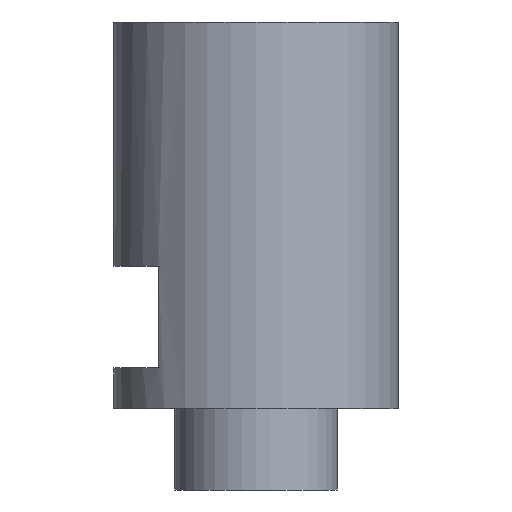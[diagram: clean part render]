
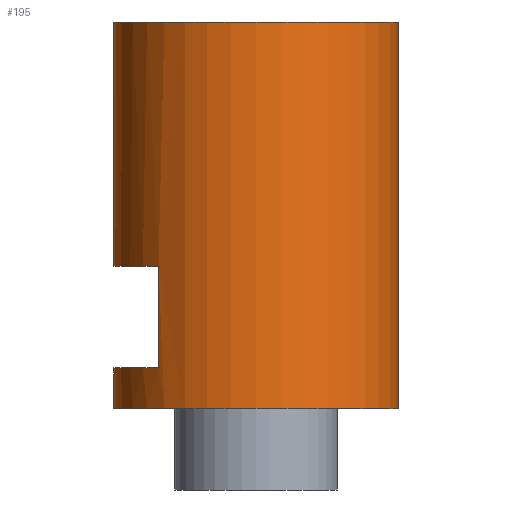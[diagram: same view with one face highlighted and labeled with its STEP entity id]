
A CAD part, front view. The second image highlights one B-rep face of the part: STEP entity #195.
In plain terms, the highlighted cylindrical face has radius 7 mm (diameter 14 mm), a partial arc.
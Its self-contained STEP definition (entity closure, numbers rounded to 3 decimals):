
#3 = CIRCLE ( 'NONE', #515, 7. ) ;
#4 = ORIENTED_EDGE ( 'NONE', *, *, #141, .T. ) ;
#9 = ORIENTED_EDGE ( 'NONE', *, *, #354, .F. ) ;
#28 = DIRECTION ( 'NONE',  ( 1., 0., 0. ) ) ;
#29 = CIRCLE ( 'NONE', #196, 7. ) ;
#32 = VERTEX_POINT ( 'NONE', #520 ) ;
#38 = LINE ( 'NONE', #447, #513 ) ;
#43 = DIRECTION ( 'NONE',  ( 0., 0., -1. ) ) ;
#45 = CARTESIAN_POINT ( 'NONE',  ( 0., 0., 19. ) ) ;
#50 = AXIS2_PLACEMENT_3D ( 'NONE', #122, #299, #28 ) ;
#58 = ORIENTED_EDGE ( 'NONE', *, *, #287, .T. ) ;
#71 = DIRECTION ( 'NONE',  ( 0., 0., -1. ) ) ;
#73 = DIRECTION ( 'NONE',  ( 0., 0., -1. ) ) ;
#80 = CARTESIAN_POINT ( 'NONE',  ( -7., 0., 6. ) ) ;
#88 = EDGE_CURVE ( 'NONE', #245, #32, #222, .T. ) ;
#93 = VERTEX_POINT ( 'NONE', #264 ) ;
#96 = EDGE_LOOP ( 'NONE', ( #385, #9, #58, #238, #387, #536, #4, #511 ) ) ;
#99 = FACE_OUTER_BOUND ( 'NONE', #96, .T. ) ;
#111 = VECTOR ( 'NONE', #73, 1000. ) ;
#121 = EDGE_CURVE ( 'NONE', #168, #93, #156, .T. ) ;
#122 = CARTESIAN_POINT ( 'NONE',  ( 0., 0., 7. ) ) ;
#134 = CYLINDRICAL_SURFACE ( 'NONE', #166, 7. ) ;
#141 = EDGE_CURVE ( 'NONE', #479, #410, #38, .T. ) ;
#143 = AXIS2_PLACEMENT_3D ( 'NONE', #459, #551, #228 ) ;
#156 = LINE ( 'NONE', #203, #111 ) ;
#166 = AXIS2_PLACEMENT_3D ( 'NONE', #529, #396, #581 ) ;
#168 = VERTEX_POINT ( 'NONE', #348 ) ;
#172 = VECTOR ( 'NONE', #43, 1000. ) ;
#180 = DIRECTION ( 'NONE',  ( 1., 0., 0. ) ) ;
#189 = LINE ( 'NONE', #80, #172 ) ;
#190 = DIRECTION ( 'NONE',  ( 0., 0., -1. ) ) ;
#195 = ADVANCED_FACE ( 'NONE', ( #99 ), #134, .T. ) ;
#196 = AXIS2_PLACEMENT_3D ( 'NONE', #45, #317, #180 ) ;
#203 = CARTESIAN_POINT ( 'NONE',  ( 7., 0., 6. ) ) ;
#212 = EDGE_CURVE ( 'NONE', #479, #487, #3, .T. ) ;
#222 = CIRCLE ( 'NONE', #50, 7. ) ;
#221 = CARTESIAN_POINT ( 'NONE',  ( 0., 0., 2. ) ) ;
#228 = DIRECTION ( 'NONE',  ( 1., 0., 0. ) ) ;
#238 = ORIENTED_EDGE ( 'NONE', *, *, #88, .T. ) ;
#243 = VECTOR ( 'NONE', #190, 1000. ) ;
#245 = VERTEX_POINT ( 'NONE', #266 ) ;
#264 = CARTESIAN_POINT ( 'NONE',  ( 7., 0., 0. ) ) ;
#266 = CARTESIAN_POINT ( 'NONE',  ( -7., 0., 7. ) ) ;
#269 = DIRECTION ( 'NONE',  ( 1., 0., 0. ) ) ;
#287 = EDGE_CURVE ( 'NONE', #428, #245, #189, .T. ) ;
#299 = DIRECTION ( 'NONE',  ( 0., 0., 1. ) ) ;
#311 = CARTESIAN_POINT ( 'NONE',  ( -7., 0., 0. ) ) ;
#313 = DIRECTION ( 'NONE',  ( 0., 0., 1. ) ) ;
#317 = DIRECTION ( 'NONE',  ( 0., 0., 1. ) ) ;
#337 = EDGE_CURVE ( 'NONE', #410, #93, #357, .T. ) ;
#348 = CARTESIAN_POINT ( 'NONE',  ( 7., 0., 19. ) ) ;
#354 = EDGE_CURVE ( 'NONE', #428, #168, #29, .T. ) ;
#357 = CIRCLE ( 'NONE', #143, 7. ) ;
#360 = CARTESIAN_POINT ( 'NONE',  ( -7., 0., 19. ) ) ;
#375 = CARTESIAN_POINT ( 'NONE',  ( -7., 0., 2. ) ) ;
#376 = LINE ( 'NONE', #505, #243 ) ;
#385 = ORIENTED_EDGE ( 'NONE', *, *, #121, .F. ) ;
#387 = ORIENTED_EDGE ( 'NONE', *, *, #507, .T. ) ;
#396 = DIRECTION ( 'NONE',  ( 0., 0., -1. ) ) ;
#410 = VERTEX_POINT ( 'NONE', #311 ) ;
#424 = CARTESIAN_POINT ( 'NONE',  ( -4.795, -5.1, 2. ) ) ;
#428 = VERTEX_POINT ( 'NONE', #360 ) ;
#447 = CARTESIAN_POINT ( 'NONE',  ( -7., 0., 6. ) ) ;
#459 = CARTESIAN_POINT ( 'NONE',  ( 0., 0., 0. ) ) ;
#479 = VERTEX_POINT ( 'NONE', #375 ) ;
#487 = VERTEX_POINT ( 'NONE', #424 ) ;
#505 = CARTESIAN_POINT ( 'NONE',  ( -4.795, -5.1, 6. ) ) ;
#507 = EDGE_CURVE ( 'NONE', #32, #487, #376, .T. ) ;
#511 = ORIENTED_EDGE ( 'NONE', *, *, #337, .T. ) ;
#513 = VECTOR ( 'NONE', #71, 1000. ) ;
#515 = AXIS2_PLACEMENT_3D ( 'NONE', #221, #313, #269 ) ;
#520 = CARTESIAN_POINT ( 'NONE',  ( -4.795, -5.1, 7. ) ) ;
#529 = CARTESIAN_POINT ( 'NONE',  ( 0., 0., 6. ) ) ;
#536 = ORIENTED_EDGE ( 'NONE', *, *, #212, .F. ) ;
#551 = DIRECTION ( 'NONE',  ( 0., 0., 1. ) ) ;
#581 = DIRECTION ( 'NONE',  ( -1., 0., 0. ) ) ;
